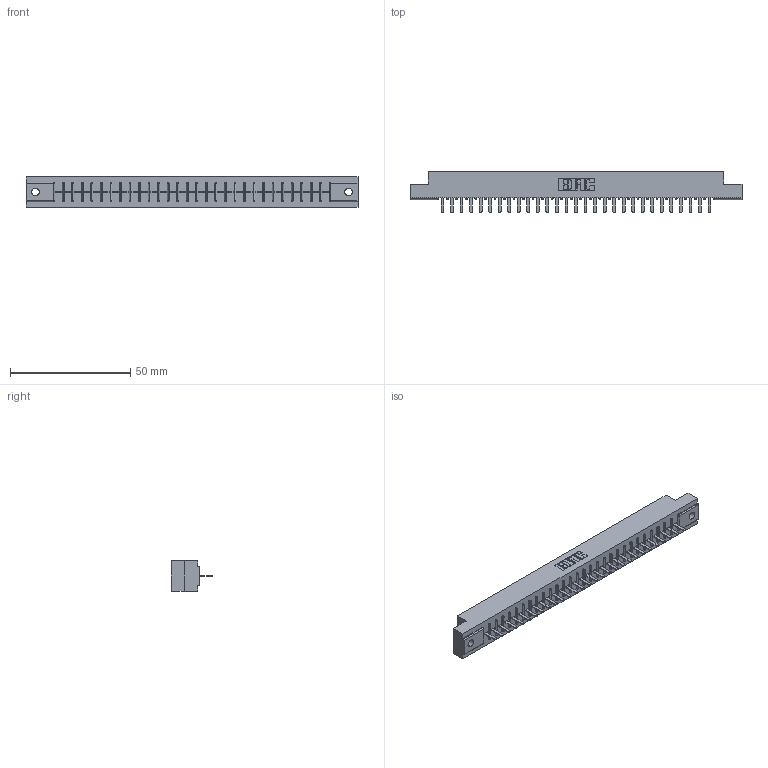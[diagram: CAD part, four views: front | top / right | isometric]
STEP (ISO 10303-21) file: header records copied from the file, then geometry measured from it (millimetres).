
FILE_DESCRIPTION (( 'STEP AP203' ), '1' );
FILE_NAME ('356-029-420-102.STEP', '2020-09-23T18:58:05', ( '' ), ( '' ), 'SwSTEP 2.0', 'SolidWorks 2020', '' );
FILE_SCHEMA (( 'CONFIG_CONTROL_DESIGN' ));
Length unit declared in the file: inch
Products named in the file (3): 306-290-001_120; 306 Part_.128 Dia; 356-029-420-102
Assembly tree (30 placements, depth 2):
  356-029-420-102
    306 Part_.128 Dia
    306-290-001_120  x29
Bounding box: 137.92 x 17.12 x 12.7 mm (x, y, z)
Volume: 15098.4 mm3; surface area: 15096.8 mm2
Topology: 30 solids, 30 shells, 2146 faces, 6029 edges, 3862 vertices
Faces by surface type: plane 1431, cylinder 599, sphere 116
Entity records: 28686 total; most frequent: CARTESIAN_POINT 4814, ORIENTED_EDGE 4770, DIRECTION 4749, EDGE_CURVE 2385, VECTOR 1859, LINE 1859, VERTEX_POINT 1510, AXIS2_PLACEMENT_3D 1445
